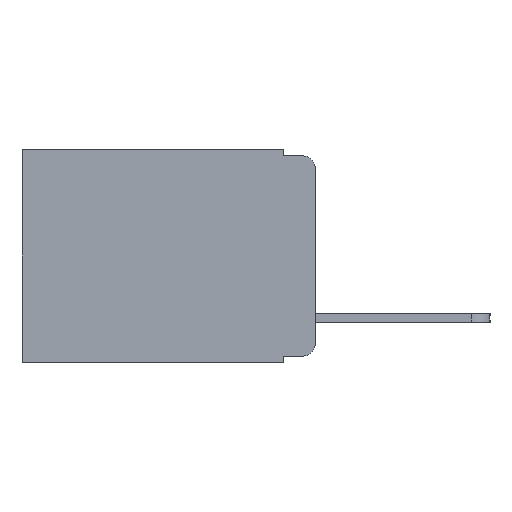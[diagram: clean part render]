
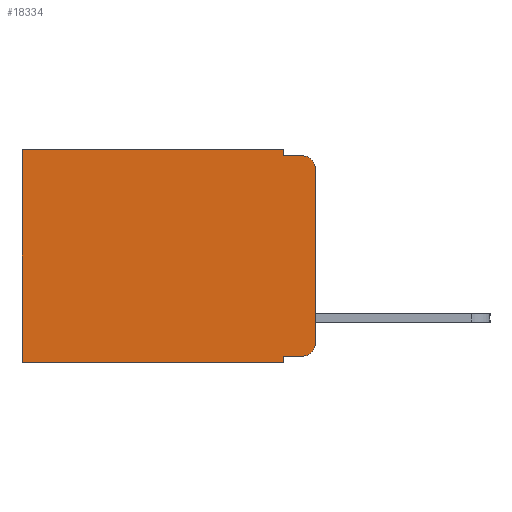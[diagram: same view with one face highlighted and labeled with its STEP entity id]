
A CAD part, left-side view. The second image highlights one B-rep face of the part: STEP entity #18334.
In plain terms, the highlighted planar face has unit normal (-1, 0, 0).
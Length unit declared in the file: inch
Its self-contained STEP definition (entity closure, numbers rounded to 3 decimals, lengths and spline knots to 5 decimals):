
#425 = VECTOR ( 'NONE', #20696, 39.37008 ) ;
#436 = DIRECTION ( 'NONE',  ( 0., 0., -1. ) ) ;
#560 = LINE ( 'NONE', #7177, #17342 ) ;
#676 = VECTOR ( 'NONE', #13718, 39.37008 ) ;
#844 = DIRECTION ( 'NONE',  ( 0., 0., -1. ) ) ;
#1164 = LINE ( 'NONE', #1335, #14198 ) ;
#1246 = AXIS2_PLACEMENT_3D ( 'NONE', #19680, #10515, #436 ) ;
#1335 = CARTESIAN_POINT ( 'NONE',  ( 0.298, 0.051, 0. ) ) ;
#1795 = EDGE_CURVE ( 'NONE', #11665, #1984, #6538, .T. ) ;
#1874 = CARTESIAN_POINT ( 'NONE',  ( 0.298, 0.02, -0.313 ) ) ;
#1984 = VERTEX_POINT ( 'NONE', #19872 ) ;
#2135 = EDGE_CURVE ( 'NONE', #18429, #5404, #5512, .T. ) ;
#2249 = ORIENTED_EDGE ( 'NONE', *, *, #14876, .T. ) ;
#2531 = AXIS2_PLACEMENT_3D ( 'NONE', #17015, #10834, #844 ) ;
#2565 = ORIENTED_EDGE ( 'NONE', *, *, #2135, .F. ) ;
#3277 = ORIENTED_EDGE ( 'NONE', *, *, #1795, .T. ) ;
#3600 = CARTESIAN_POINT ( 'NONE',  ( 0.298, 0.051, -0.01 ) ) ;
#3834 = VERTEX_POINT ( 'NONE', #7794 ) ;
#3868 = CARTESIAN_POINT ( 'NONE',  ( 0.298, 0.051, 0. ) ) ;
#4416 = AXIS2_PLACEMENT_3D ( 'NONE', #1874, #5022, #9753 ) ;
#4494 = PLANE ( 'NONE',  #2531 ) ;
#4588 = ORIENTED_EDGE ( 'NONE', *, *, #10745, .F. ) ;
#4606 = EDGE_CURVE ( 'NONE', #6331, #9854, #7558, .T. ) ;
#4756 = LINE ( 'NONE', #17346, #425 ) ;
#4999 = CARTESIAN_POINT ( 'NONE',  ( 0.298, 0.051, -0.333 ) ) ;
#5022 = DIRECTION ( 'NONE',  ( -1., 0., 0. ) ) ;
#5404 = VERTEX_POINT ( 'NONE', #19435 ) ;
#5512 = LINE ( 'NONE', #9206, #676 ) ;
#5536 = CARTESIAN_POINT ( 'NONE',  ( 0.298, 0., -0.03 ) ) ;
#5583 = DIRECTION ( 'NONE',  ( 0., 0., -1. ) ) ;
#6242 = EDGE_CURVE ( 'NONE', #3834, #8639, #4756, .T. ) ;
#6331 = VERTEX_POINT ( 'NONE', #5536 ) ;
#6407 = ORIENTED_EDGE ( 'NONE', *, *, #13518, .F. ) ;
#6538 = LINE ( 'NONE', #12564, #14299 ) ;
#7177 = CARTESIAN_POINT ( 'NONE',  ( 0.298, 0.473, 0. ) ) ;
#7558 = LINE ( 'NONE', #10826, #18923 ) ;
#7794 = CARTESIAN_POINT ( 'NONE',  ( 0.298, 0.051, 0. ) ) ;
#7820 = ORIENTED_EDGE ( 'NONE', *, *, #4606, .F. ) ;
#8639 = VERTEX_POINT ( 'NONE', #20572 ) ;
#8664 = DIRECTION ( 'NONE',  ( 0., 0., -1. ) ) ;
#9082 = CIRCLE ( 'NONE', #4416, 0.02 ) ;
#9206 = CARTESIAN_POINT ( 'NONE',  ( 0.298, 0., -0.343 ) ) ;
#9353 = CARTESIAN_POINT ( 'NONE',  ( 0.298, 0.051, -0.01 ) ) ;
#9435 = DIRECTION ( 'NONE',  ( 0., 0., -1. ) ) ;
#9753 = DIRECTION ( 'NONE',  ( 0., 0., -1. ) ) ;
#9757 = CIRCLE ( 'NONE', #1246, 0.02 ) ;
#9854 = VERTEX_POINT ( 'NONE', #16171 ) ;
#10032 = FACE_OUTER_BOUND ( 'NONE', #11401, .T. ) ;
#10389 = EDGE_CURVE ( 'NONE', #8639, #5404, #560, .T. ) ;
#10515 = DIRECTION ( 'NONE',  ( -1., 0., 0. ) ) ;
#10745 = EDGE_CURVE ( 'NONE', #18318, #13055, #18516, .T. ) ;
#10826 = CARTESIAN_POINT ( 'NONE',  ( 0.298, 0., 0. ) ) ;
#10834 = DIRECTION ( 'NONE',  ( 1., 0., 0. ) ) ;
#11401 = EDGE_LOOP ( 'NONE', ( #7820, #20553, #4588, #20776, #17314, #16737, #2565, #6407, #3277, #2249 ) ) ;
#11665 = VERTEX_POINT ( 'NONE', #4999 ) ;
#12564 = CARTESIAN_POINT ( 'NONE',  ( 0.298, 0.051, -0.333 ) ) ;
#12601 = CARTESIAN_POINT ( 'NONE',  ( 0.298, 0.051, -0.343 ) ) ;
#13055 = VERTEX_POINT ( 'NONE', #17578 ) ;
#13518 = EDGE_CURVE ( 'NONE', #11665, #18429, #1164, .T. ) ;
#13670 = DIRECTION ( 'NONE',  ( 0., -1., 0. ) ) ;
#13718 = DIRECTION ( 'NONE',  ( 0., 1., 0. ) ) ;
#14114 = LINE ( 'NONE', #3868, #17743 ) ;
#14198 = VECTOR ( 'NONE', #14352, 39.37008 ) ;
#14222 = DIRECTION ( 'NONE',  ( 0., -1., 0. ) ) ;
#14299 = VECTOR ( 'NONE', #14222, 39.37008 ) ;
#14352 = DIRECTION ( 'NONE',  ( 0., 0., -1. ) ) ;
#14413 = VECTOR ( 'NONE', #13670, 39.37008 ) ;
#14876 = EDGE_CURVE ( 'NONE', #1984, #9854, #9082, .T. ) ;
#16171 = CARTESIAN_POINT ( 'NONE',  ( 0.298, 0., -0.313 ) ) ;
#16737 = ORIENTED_EDGE ( 'NONE', *, *, #10389, .T. ) ;
#17015 = CARTESIAN_POINT ( 'NONE',  ( 0.298, 0., 0. ) ) ;
#17314 = ORIENTED_EDGE ( 'NONE', *, *, #6242, .T. ) ;
#17342 = VECTOR ( 'NONE', #9435, 39.37008 ) ;
#17346 = CARTESIAN_POINT ( 'NONE',  ( 0.298, 0., 0. ) ) ;
#17578 = CARTESIAN_POINT ( 'NONE',  ( 0.298, 0.02, -0.01 ) ) ;
#17743 = VECTOR ( 'NONE', #5583, 39.37008 ) ;
#18318 = VERTEX_POINT ( 'NONE', #3600 ) ;
#18334 = ADVANCED_FACE ( 'NONE', ( #10032 ), #4494, .F. ) ;
#18429 = VERTEX_POINT ( 'NONE', #12601 ) ;
#18516 = LINE ( 'NONE', #9353, #14413 ) ;
#18637 = EDGE_CURVE ( 'NONE', #3834, #18318, #14114, .T. ) ;
#18923 = VECTOR ( 'NONE', #8664, 39.37008 ) ;
#19435 = CARTESIAN_POINT ( 'NONE',  ( 0.298, 0.473, -0.343 ) ) ;
#19680 = CARTESIAN_POINT ( 'NONE',  ( 0.298, 0.02, -0.03 ) ) ;
#19869 = EDGE_CURVE ( 'NONE', #6331, #13055, #9757, .T. ) ;
#19872 = CARTESIAN_POINT ( 'NONE',  ( 0.298, 0.02, -0.333 ) ) ;
#20553 = ORIENTED_EDGE ( 'NONE', *, *, #19869, .T. ) ;
#20572 = CARTESIAN_POINT ( 'NONE',  ( 0.298, 0.473, 0. ) ) ;
#20696 = DIRECTION ( 'NONE',  ( 0., 1., 0. ) ) ;
#20776 = ORIENTED_EDGE ( 'NONE', *, *, #18637, .F. ) ;
